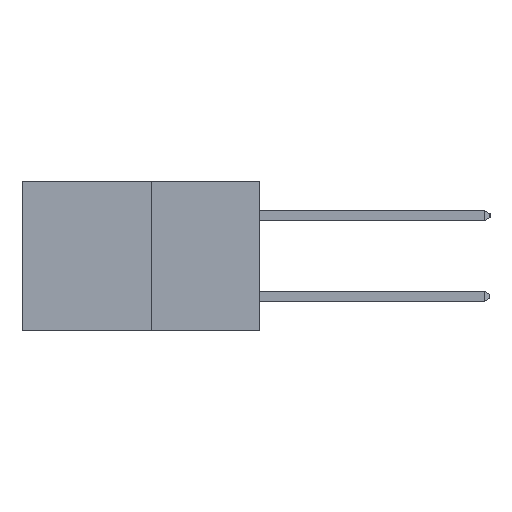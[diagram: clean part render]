
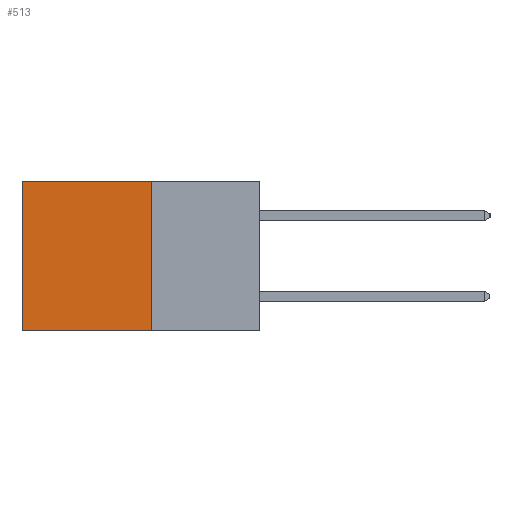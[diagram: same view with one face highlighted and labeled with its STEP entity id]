
A CAD part, left-side view. The second image highlights one B-rep face of the part: STEP entity #513.
In plain terms, the highlighted planar face has unit normal (-1, 0, 0).
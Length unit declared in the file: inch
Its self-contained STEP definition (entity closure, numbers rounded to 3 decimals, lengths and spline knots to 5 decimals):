
#41 = CARTESIAN_POINT ( 'NONE',  ( 0.277, 0.27, -0.37 ) ) ;
#513 = ADVANCED_FACE ( 'NONE', ( #10329 ), #6538, .F. ) ;
#1889 = LINE ( 'NONE', #10586, #13248 ) ;
#2224 = CARTESIAN_POINT ( 'NONE',  ( 0.277, 0.27, 0. ) ) ;
#2650 = EDGE_CURVE ( 'NONE', #3568, #3246, #10099, .T. ) ;
#2707 = VERTEX_POINT ( 'NONE', #14182 ) ;
#3209 = CARTESIAN_POINT ( 'NONE',  ( 0.277, 0.59, 0. ) ) ;
#3246 = VERTEX_POINT ( 'NONE', #3706 ) ;
#3568 = VERTEX_POINT ( 'NONE', #3209 ) ;
#3706 = CARTESIAN_POINT ( 'NONE',  ( 0.277, 0.59, -0.37 ) ) ;
#3982 = EDGE_CURVE ( 'NONE', #2707, #3246, #1889, .T. ) ;
#4123 = EDGE_LOOP ( 'NONE', ( #12457, #14083, #6708, #10408 ) ) ;
#4176 = AXIS2_PLACEMENT_3D ( 'NONE', #5237, #5464, #4355 ) ;
#4355 = DIRECTION ( 'NONE',  ( 0., 0., -1. ) ) ;
#4770 = LINE ( 'NONE', #41, #10324 ) ;
#4796 = VECTOR ( 'NONE', #13985, 39.37008 ) ;
#5237 = CARTESIAN_POINT ( 'NONE',  ( 0.277, 0.27, -0.37 ) ) ;
#5464 = DIRECTION ( 'NONE',  ( 1., 0., 0. ) ) ;
#5491 = LINE ( 'NONE', #8678, #4796 ) ;
#6538 = PLANE ( 'NONE',  #4176 ) ;
#6708 = ORIENTED_EDGE ( 'NONE', *, *, #10242, .F. ) ;
#6730 = DIRECTION ( 'NONE',  ( 0., 0., -1. ) ) ;
#7271 = VERTEX_POINT ( 'NONE', #2224 ) ;
#7360 = DIRECTION ( 'NONE',  ( 0., 0., -1. ) ) ;
#8678 = CARTESIAN_POINT ( 'NONE',  ( 0.277, 0.27, 0. ) ) ;
#9384 = EDGE_CURVE ( 'NONE', #7271, #3568, #5491, .T. ) ;
#10099 = LINE ( 'NONE', #12072, #12638 ) ;
#10242 = EDGE_CURVE ( 'NONE', #7271, #2707, #4770, .T. ) ;
#10324 = VECTOR ( 'NONE', #6730, 39.37008 ) ;
#10329 = FACE_OUTER_BOUND ( 'NONE', #4123, .T. ) ;
#10408 = ORIENTED_EDGE ( 'NONE', *, *, #9384, .T. ) ;
#10586 = CARTESIAN_POINT ( 'NONE',  ( 0.277, 0.27, -0.37 ) ) ;
#10770 = DIRECTION ( 'NONE',  ( 0., 1., 0. ) ) ;
#12072 = CARTESIAN_POINT ( 'NONE',  ( 0.277, 0.59, -0.37 ) ) ;
#12457 = ORIENTED_EDGE ( 'NONE', *, *, #2650, .T. ) ;
#12638 = VECTOR ( 'NONE', #7360, 39.37008 ) ;
#13248 = VECTOR ( 'NONE', #10770, 39.37008 ) ;
#13985 = DIRECTION ( 'NONE',  ( 0., 1., 0. ) ) ;
#14083 = ORIENTED_EDGE ( 'NONE', *, *, #3982, .F. ) ;
#14182 = CARTESIAN_POINT ( 'NONE',  ( 0.277, 0.27, -0.37 ) ) ;
